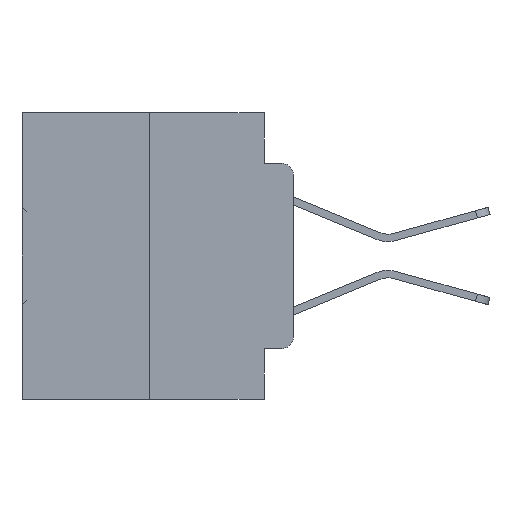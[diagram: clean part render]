
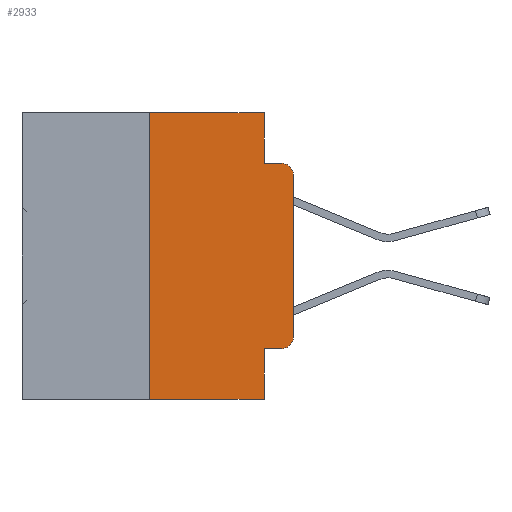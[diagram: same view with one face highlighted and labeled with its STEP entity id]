
A CAD part, left-side view. The second image highlights one B-rep face of the part: STEP entity #2933.
In plain terms, the highlighted planar face has unit normal (-1, 0, 0).
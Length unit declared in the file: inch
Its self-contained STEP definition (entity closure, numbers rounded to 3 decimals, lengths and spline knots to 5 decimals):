
#730 = VERTEX_POINT ( 'NONE', #25185 ) ;
#775 = CARTESIAN_POINT ( 'NONE',  ( 0., 0.051, 0. ) ) ;
#1337 = VECTOR ( 'NONE', #7162, 39.37008 ) ;
#2047 = VERTEX_POINT ( 'NONE', #33138 ) ;
#2172 = CARTESIAN_POINT ( 'NONE',  ( 0., 0.473, 0. ) ) ;
#2478 = DIRECTION ( 'NONE',  ( -1., 0., 0. ) ) ;
#2933 = ADVANCED_FACE ( 'NONE', ( #8143 ), #5316, .F. ) ;
#3039 = VECTOR ( 'NONE', #11782, 39.37008 ) ;
#3492 = CARTESIAN_POINT ( 'NONE',  ( 0., 0.02, -0.1085 ) ) ;
#3913 = LINE ( 'NONE', #20228, #3039 ) ;
#3943 = CARTESIAN_POINT ( 'NONE',  ( 0., 0.051, -0.0885 ) ) ;
#5093 = CARTESIAN_POINT ( 'NONE',  ( 0., 0.02, -0.4115 ) ) ;
#5316 = PLANE ( 'NONE',  #20837 ) ;
#5327 = EDGE_CURVE ( 'NONE', #15453, #2047, #11166, .T. ) ;
#6621 = AXIS2_PLACEMENT_3D ( 'NONE', #3492, #28967, #17336 ) ;
#6986 = LINE ( 'NONE', #8385, #29816 ) ;
#7162 = DIRECTION ( 'NONE',  ( 0., -1., 0. ) ) ;
#7386 = DIRECTION ( 'NONE',  ( 0., 0., 1. ) ) ;
#7637 = EDGE_CURVE ( 'NONE', #35942, #2047, #11822, .T. ) ;
#8052 = EDGE_CURVE ( 'NONE', #35942, #29380, #3913, .T. ) ;
#8143 = FACE_OUTER_BOUND ( 'NONE', #19556, .T. ) ;
#8385 = CARTESIAN_POINT ( 'NONE',  ( 0., 0.051, -0.0885 ) ) ;
#8976 = ORIENTED_EDGE ( 'NONE', *, *, #19180, .T. ) ;
#9780 = CIRCLE ( 'NONE', #24180, 0.02 ) ;
#9850 = EDGE_CURVE ( 'NONE', #15453, #11705, #16053, .T. ) ;
#10617 = DIRECTION ( 'NONE',  ( 0., 0., -1. ) ) ;
#11166 = LINE ( 'NONE', #21291, #19498 ) ;
#11228 = CARTESIAN_POINT ( 'NONE',  ( 0., 0.25, -0.5 ) ) ;
#11705 = VERTEX_POINT ( 'NONE', #5093 ) ;
#11782 = DIRECTION ( 'NONE',  ( 0., 0., 1. ) ) ;
#11822 = LINE ( 'NONE', #29334, #1337 ) ;
#11823 = VECTOR ( 'NONE', #7386, 39.37008 ) ;
#11974 = EDGE_CURVE ( 'NONE', #25599, #730, #6986, .T. ) ;
#12470 = ORIENTED_EDGE ( 'NONE', *, *, #33881, .T. ) ;
#12660 = CARTESIAN_POINT ( 'NONE',  ( 0., 0., 0. ) ) ;
#12667 = CARTESIAN_POINT ( 'NONE',  ( 0., 0.25, 0. ) ) ;
#13367 = CARTESIAN_POINT ( 'NONE',  ( 0., 0.02, -0.3915 ) ) ;
#13596 = LINE ( 'NONE', #12660, #11823 ) ;
#14718 = LINE ( 'NONE', #775, #15134 ) ;
#14746 = VECTOR ( 'NONE', #18706, 39.37008 ) ;
#14886 = CARTESIAN_POINT ( 'NONE',  ( 0., 0., -0.1085 ) ) ;
#15134 = VECTOR ( 'NONE', #34499, 39.37008 ) ;
#15350 = CARTESIAN_POINT ( 'NONE',  ( 0., 0.051, -0.4115 ) ) ;
#15453 = VERTEX_POINT ( 'NONE', #15350 ) ;
#15496 = LINE ( 'NONE', #35701, #25994 ) ;
#16053 = LINE ( 'NONE', #24592, #14746 ) ;
#16759 = CARTESIAN_POINT ( 'NONE',  ( 0., 0.051, 0. ) ) ;
#17225 = VERTEX_POINT ( 'NONE', #16759 ) ;
#17336 = DIRECTION ( 'NONE',  ( 0., 0., -1. ) ) ;
#18706 = DIRECTION ( 'NONE',  ( 0., -1., 0. ) ) ;
#18866 = ORIENTED_EDGE ( 'NONE', *, *, #8052, .F. ) ;
#18908 = EDGE_CURVE ( 'NONE', #29380, #17225, #15496, .T. ) ;
#19180 = EDGE_CURVE ( 'NONE', #34310, #730, #33450, .T. ) ;
#19498 = VECTOR ( 'NONE', #35655, 39.37008 ) ;
#19556 = EDGE_LOOP ( 'NONE', ( #12470, #8976, #26147, #24154, #23590, #18866, #24607, #23345, #35653, #29372 ) ) ;
#19782 = DIRECTION ( 'NONE',  ( 0., -1., 0. ) ) ;
#20228 = CARTESIAN_POINT ( 'NONE',  ( 0., 0.25, 0. ) ) ;
#20837 = AXIS2_PLACEMENT_3D ( 'NONE', #2172, #24588, #10617 ) ;
#21213 = DIRECTION ( 'NONE',  ( 0., -1., 0. ) ) ;
#21291 = CARTESIAN_POINT ( 'NONE',  ( 0., 0.051, 0. ) ) ;
#22247 = EDGE_CURVE ( 'NONE', #17225, #25599, #14718, .T. ) ;
#23345 = ORIENTED_EDGE ( 'NONE', *, *, #5327, .F. ) ;
#23590 = ORIENTED_EDGE ( 'NONE', *, *, #18908, .F. ) ;
#24154 = ORIENTED_EDGE ( 'NONE', *, *, #22247, .F. ) ;
#24180 = AXIS2_PLACEMENT_3D ( 'NONE', #13367, #2478, #30022 ) ;
#24588 = DIRECTION ( 'NONE',  ( 1., 0., 0. ) ) ;
#24592 = CARTESIAN_POINT ( 'NONE',  ( 0., 0.051, -0.4115 ) ) ;
#24607 = ORIENTED_EDGE ( 'NONE', *, *, #7637, .T. ) ;
#25185 = CARTESIAN_POINT ( 'NONE',  ( 0., 0.02, -0.0885 ) ) ;
#25599 = VERTEX_POINT ( 'NONE', #3943 ) ;
#25994 = VECTOR ( 'NONE', #21213, 39.37008 ) ;
#26147 = ORIENTED_EDGE ( 'NONE', *, *, #11974, .F. ) ;
#28967 = DIRECTION ( 'NONE',  ( -1., 0., 0. ) ) ;
#29096 = VERTEX_POINT ( 'NONE', #31290 ) ;
#29334 = CARTESIAN_POINT ( 'NONE',  ( 0., 0.473, -0.5 ) ) ;
#29372 = ORIENTED_EDGE ( 'NONE', *, *, #30553, .T. ) ;
#29380 = VERTEX_POINT ( 'NONE', #12667 ) ;
#29816 = VECTOR ( 'NONE', #19782, 39.37008 ) ;
#30022 = DIRECTION ( 'NONE',  ( 0., 0., -1. ) ) ;
#30553 = EDGE_CURVE ( 'NONE', #11705, #29096, #9780, .T. ) ;
#31290 = CARTESIAN_POINT ( 'NONE',  ( 0., 0., -0.3915 ) ) ;
#33138 = CARTESIAN_POINT ( 'NONE',  ( 0., 0.051, -0.5 ) ) ;
#33450 = CIRCLE ( 'NONE', #6621, 0.02 ) ;
#33881 = EDGE_CURVE ( 'NONE', #29096, #34310, #13596, .T. ) ;
#34310 = VERTEX_POINT ( 'NONE', #14886 ) ;
#34499 = DIRECTION ( 'NONE',  ( 0., 0., -1. ) ) ;
#35653 = ORIENTED_EDGE ( 'NONE', *, *, #9850, .T. ) ;
#35655 = DIRECTION ( 'NONE',  ( 0., 0., -1. ) ) ;
#35701 = CARTESIAN_POINT ( 'NONE',  ( 0., 0.473, 0. ) ) ;
#35942 = VERTEX_POINT ( 'NONE', #11228 ) ;
